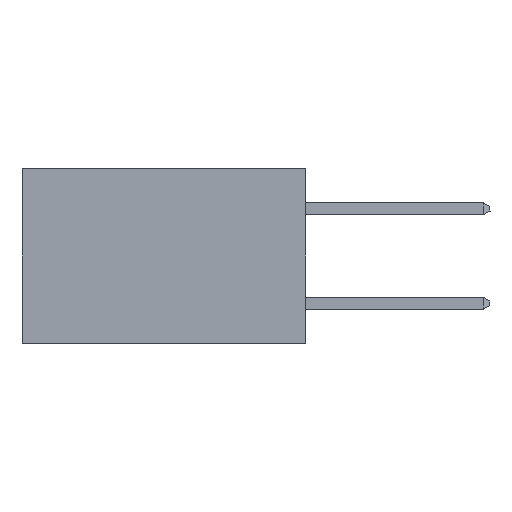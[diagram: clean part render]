
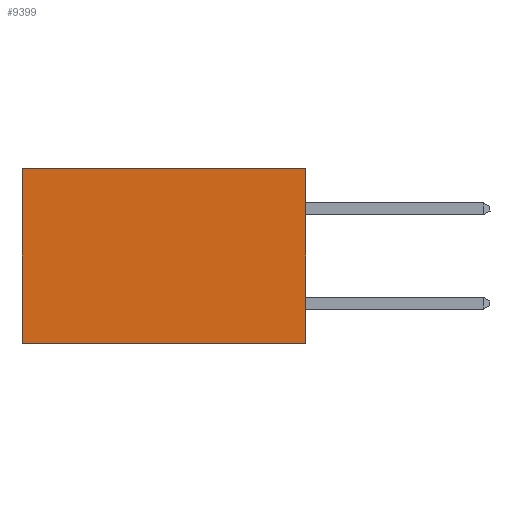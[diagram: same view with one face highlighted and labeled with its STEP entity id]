
A CAD part, left-side view. The second image highlights one B-rep face of the part: STEP entity #9399.
In plain terms, the highlighted planar face has unit normal (-1, 0, 0).
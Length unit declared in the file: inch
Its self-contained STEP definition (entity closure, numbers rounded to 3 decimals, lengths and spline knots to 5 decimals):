
#44 = EDGE_LOOP ( 'NONE', ( #12450, #11587, #5178, #6114 ) ) ;
#723 = CARTESIAN_POINT ( 'NONE',  ( 0.298, 0., -0.37 ) ) ;
#1213 = CARTESIAN_POINT ( 'NONE',  ( 0.298, 0.6, 0. ) ) ;
#1466 = CARTESIAN_POINT ( 'NONE',  ( 0.298, 0.6, 0. ) ) ;
#2785 = CARTESIAN_POINT ( 'NONE',  ( 0.298, 0., 0. ) ) ;
#2832 = DIRECTION ( 'NONE',  ( 1., 0., 0. ) ) ;
#3181 = VECTOR ( 'NONE', #12053, 39.37008 ) ;
#3293 = EDGE_CURVE ( 'NONE', #3753, #10030, #9380, .T. ) ;
#3462 = AXIS2_PLACEMENT_3D ( 'NONE', #2785, #2832, #9116 ) ;
#3506 = VECTOR ( 'NONE', #4884, 39.37008 ) ;
#3753 = VERTEX_POINT ( 'NONE', #5764 ) ;
#3849 = LINE ( 'NONE', #1466, #3181 ) ;
#3937 = PLANE ( 'NONE',  #3462 ) ;
#4512 = VERTEX_POINT ( 'NONE', #1213 ) ;
#4884 = DIRECTION ( 'NONE',  ( 0., 0., -1. ) ) ;
#5178 = ORIENTED_EDGE ( 'NONE', *, *, #12742, .F. ) ;
#5303 = VECTOR ( 'NONE', #9682, 39.37008 ) ;
#5764 = CARTESIAN_POINT ( 'NONE',  ( 0.298, 0., -0.37 ) ) ;
#6114 = ORIENTED_EDGE ( 'NONE', *, *, #13467, .T. ) ;
#8454 = CARTESIAN_POINT ( 'NONE',  ( 0.298, 0., 0. ) ) ;
#8560 = CARTESIAN_POINT ( 'NONE',  ( 0.298, 0., 0. ) ) ;
#9116 = DIRECTION ( 'NONE',  ( 0., 0., -1. ) ) ;
#9380 = LINE ( 'NONE', #723, #10336 ) ;
#9399 = ADVANCED_FACE ( 'NONE', ( #9865 ), #3937, .F. ) ;
#9682 = DIRECTION ( 'NONE',  ( 0., 1., 0. ) ) ;
#9865 = FACE_OUTER_BOUND ( 'NONE', #44, .T. ) ;
#10030 = VERTEX_POINT ( 'NONE', #10603 ) ;
#10336 = VECTOR ( 'NONE', #12147, 39.37008 ) ;
#10409 = LINE ( 'NONE', #13221, #3506 ) ;
#10571 = LINE ( 'NONE', #8560, #5303 ) ;
#10603 = CARTESIAN_POINT ( 'NONE',  ( 0.298, 0.6, -0.37 ) ) ;
#11175 = VERTEX_POINT ( 'NONE', #8454 ) ;
#11587 = ORIENTED_EDGE ( 'NONE', *, *, #3293, .F. ) ;
#12053 = DIRECTION ( 'NONE',  ( 0., 0., -1. ) ) ;
#12147 = DIRECTION ( 'NONE',  ( 0., 1., 0. ) ) ;
#12450 = ORIENTED_EDGE ( 'NONE', *, *, #12592, .T. ) ;
#12592 = EDGE_CURVE ( 'NONE', #4512, #10030, #3849, .T. ) ;
#12742 = EDGE_CURVE ( 'NONE', #11175, #3753, #10409, .T. ) ;
#13221 = CARTESIAN_POINT ( 'NONE',  ( 0.298, 0., 0. ) ) ;
#13467 = EDGE_CURVE ( 'NONE', #11175, #4512, #10571, .T. ) ;
